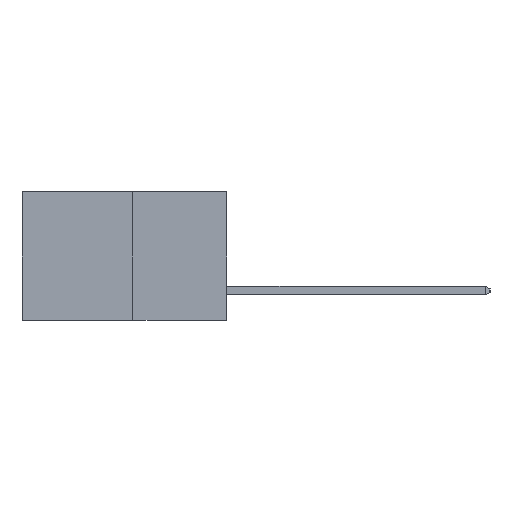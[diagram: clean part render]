
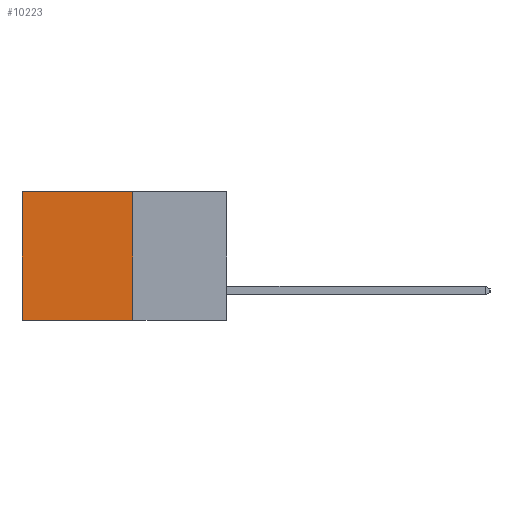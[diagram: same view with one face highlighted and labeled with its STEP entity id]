
A CAD part, left-side view. The second image highlights one B-rep face of the part: STEP entity #10223.
In plain terms, the highlighted planar face has unit normal (-1, 0, 0).
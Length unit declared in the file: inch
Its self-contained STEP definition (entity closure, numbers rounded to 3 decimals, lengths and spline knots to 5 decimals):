
#253 = DIRECTION ( 'NONE',  ( 0., 0., -1. ) ) ;
#526 = DIRECTION ( 'NONE',  ( 0., 1., 0. ) ) ;
#757 = CARTESIAN_POINT ( 'NONE',  ( 0.277, 0.59, 0. ) ) ;
#806 = DIRECTION ( 'NONE',  ( 0., 1., 0. ) ) ;
#868 = CARTESIAN_POINT ( 'NONE',  ( 0.277, 0.27, 0. ) ) ;
#1312 = FACE_OUTER_BOUND ( 'NONE', #9911, .T. ) ;
#1552 = EDGE_CURVE ( 'NONE', #9524, #11235, #10646, .T. ) ;
#2012 = CARTESIAN_POINT ( 'NONE',  ( 0.277, 0.27, -0.37 ) ) ;
#2558 = VECTOR ( 'NONE', #526, 39.37008 ) ;
#2759 = LINE ( 'NONE', #7565, #2558 ) ;
#3625 = ORIENTED_EDGE ( 'NONE', *, *, #4642, .T. ) ;
#4036 = EDGE_CURVE ( 'NONE', #9524, #14138, #2759, .T. ) ;
#4345 = CARTESIAN_POINT ( 'NONE',  ( 0.277, 0.27, -0.37 ) ) ;
#4454 = VECTOR ( 'NONE', #12862, 39.37008 ) ;
#4603 = ORIENTED_EDGE ( 'NONE', *, *, #6761, .F. ) ;
#4642 = EDGE_CURVE ( 'NONE', #14138, #7363, #10399, .T. ) ;
#4972 = PLANE ( 'NONE',  #9085 ) ;
#5172 = CARTESIAN_POINT ( 'NONE',  ( 0.277, 0.59, -0.37 ) ) ;
#6054 = LINE ( 'NONE', #4345, #11578 ) ;
#6761 = EDGE_CURVE ( 'NONE', #11235, #7363, #6054, .T. ) ;
#7306 = DIRECTION ( 'NONE',  ( 1., 0., 0. ) ) ;
#7363 = VERTEX_POINT ( 'NONE', #8490 ) ;
#7565 = CARTESIAN_POINT ( 'NONE',  ( 0.277, 0.27, 0. ) ) ;
#7802 = VECTOR ( 'NONE', #11702, 39.37008 ) ;
#8490 = CARTESIAN_POINT ( 'NONE',  ( 0.277, 0.59, -0.37 ) ) ;
#9085 = AXIS2_PLACEMENT_3D ( 'NONE', #13736, #7306, #253 ) ;
#9524 = VERTEX_POINT ( 'NONE', #868 ) ;
#9911 = EDGE_LOOP ( 'NONE', ( #3625, #4603, #12029, #13764 ) ) ;
#10223 = ADVANCED_FACE ( 'NONE', ( #1312 ), #4972, .F. ) ;
#10399 = LINE ( 'NONE', #5172, #4454 ) ;
#10646 = LINE ( 'NONE', #14452, #7802 ) ;
#11235 = VERTEX_POINT ( 'NONE', #2012 ) ;
#11578 = VECTOR ( 'NONE', #806, 39.37008 ) ;
#11702 = DIRECTION ( 'NONE',  ( 0., 0., -1. ) ) ;
#12029 = ORIENTED_EDGE ( 'NONE', *, *, #1552, .F. ) ;
#12862 = DIRECTION ( 'NONE',  ( 0., 0., -1. ) ) ;
#13736 = CARTESIAN_POINT ( 'NONE',  ( 0.277, 0.27, -0.37 ) ) ;
#13764 = ORIENTED_EDGE ( 'NONE', *, *, #4036, .T. ) ;
#14138 = VERTEX_POINT ( 'NONE', #757 ) ;
#14452 = CARTESIAN_POINT ( 'NONE',  ( 0.277, 0.27, -0.37 ) ) ;
